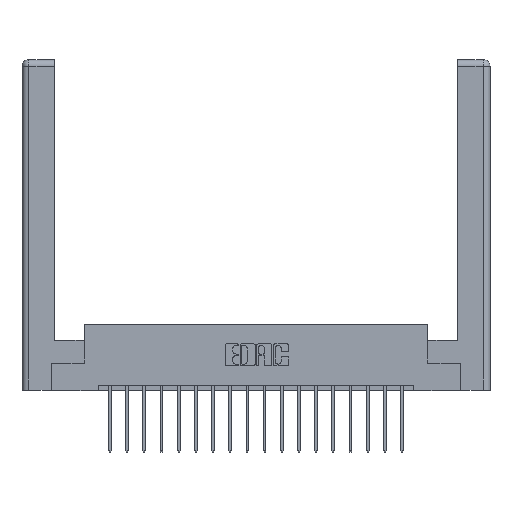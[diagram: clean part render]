
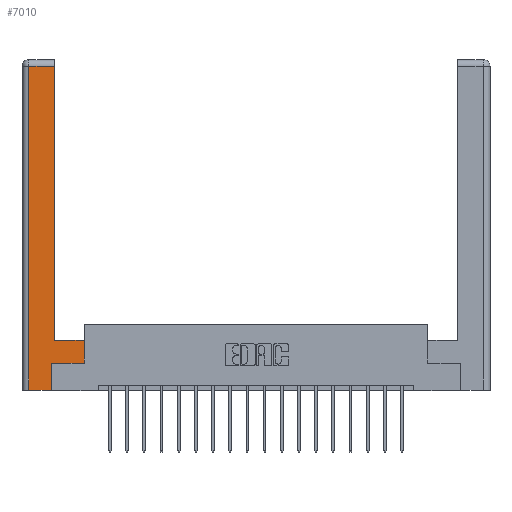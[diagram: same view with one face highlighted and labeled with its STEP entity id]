
A CAD part, top view. The second image highlights one B-rep face of the part: STEP entity #7010.
In plain terms, the highlighted planar face has unit normal (0, 0, 1).
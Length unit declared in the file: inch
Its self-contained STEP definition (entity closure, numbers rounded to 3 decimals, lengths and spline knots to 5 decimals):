
#259 = ORIENTED_EDGE ( 'NONE', *, *, #2643, .T. ) ;
#752 = DIRECTION ( 'NONE',  ( -1., 0., 0. ) ) ;
#872 = CARTESIAN_POINT ( 'NONE',  ( 0.565, 0.245, 0. ) ) ;
#1213 = VECTOR ( 'NONE', #17322, 39.37008 ) ;
#1403 = CARTESIAN_POINT ( 'NONE',  ( 0.265, 0.245, 0. ) ) ;
#1741 = LINE ( 'NONE', #13381, #9340 ) ;
#1942 = VERTEX_POINT ( 'NONE', #7242 ) ;
#1962 = EDGE_CURVE ( 'NONE', #15366, #17851, #3437, .T. ) ;
#2643 = EDGE_CURVE ( 'NONE', #3996, #12572, #1741, .T. ) ;
#3410 = LINE ( 'NONE', #872, #1213 ) ;
#3437 = LINE ( 'NONE', #14889, #15079 ) ;
#3588 = ORIENTED_EDGE ( 'NONE', *, *, #8873, .T. ) ;
#3723 = LINE ( 'NONE', #14068, #6114 ) ;
#3759 = CARTESIAN_POINT ( 'NONE',  ( 0.565, 0.245, 0. ) ) ;
#3996 = VERTEX_POINT ( 'NONE', #14719 ) ;
#5670 = ORIENTED_EDGE ( 'NONE', *, *, #1962, .T. ) ;
#5681 = LINE ( 'NONE', #6762, #17355 ) ;
#5781 = DIRECTION ( 'NONE',  ( 0., 1., 0. ) ) ;
#5881 = EDGE_CURVE ( 'NONE', #15811, #10688, #11456, .T. ) ;
#6114 = VECTOR ( 'NONE', #752, 39.37008 ) ;
#6762 = CARTESIAN_POINT ( 'NONE',  ( 0.295, 0.45, 0. ) ) ;
#6776 = CARTESIAN_POINT ( 'NONE',  ( 0.565, 0.45, 0. ) ) ;
#6832 = EDGE_CURVE ( 'NONE', #10688, #15366, #5681, .T. ) ;
#6888 = DIRECTION ( 'NONE',  ( -1., 0., 0. ) ) ;
#7006 = PLANE ( 'NONE',  #16360 ) ;
#7010 = ADVANCED_FACE ( 'NONE', ( #18062 ), #7006, .F. ) ;
#7195 = DIRECTION ( 'NONE',  ( 0., 1., 0. ) ) ;
#7242 = CARTESIAN_POINT ( 'NONE',  ( 0.265, 0.245, 0. ) ) ;
#7740 = CARTESIAN_POINT ( 'NONE',  ( 0.295, 2.94, 0. ) ) ;
#7764 = CARTESIAN_POINT ( 'NONE',  ( 0.295, 0.45, 0. ) ) ;
#8056 = EDGE_CURVE ( 'NONE', #17851, #3996, #3723, .T. ) ;
#8361 = VECTOR ( 'NONE', #18960, 39.37008 ) ;
#8441 = EDGE_LOOP ( 'NONE', ( #5670, #14473, #259, #9041, #13073, #3588, #11822, #15148 ) ) ;
#8710 = DIRECTION ( 'NONE',  ( 0., -1., 0. ) ) ;
#8873 = EDGE_CURVE ( 'NONE', #1942, #15811, #3410, .T. ) ;
#9041 = ORIENTED_EDGE ( 'NONE', *, *, #18724, .T. ) ;
#9109 = CARTESIAN_POINT ( 'NONE',  ( 0.265, 0., 0. ) ) ;
#9340 = VECTOR ( 'NONE', #8710, 39.37008 ) ;
#9548 = CARTESIAN_POINT ( 'NONE',  ( 0.0615, 0., 0. ) ) ;
#10074 = CARTESIAN_POINT ( 'NONE',  ( 0.565, 0.45, 0. ) ) ;
#10300 = DIRECTION ( 'NONE',  ( 1., 0., 0. ) ) ;
#10688 = VERTEX_POINT ( 'NONE', #10074 ) ;
#11192 = VECTOR ( 'NONE', #7195, 39.37008 ) ;
#11456 = LINE ( 'NONE', #6776, #8361 ) ;
#11822 = ORIENTED_EDGE ( 'NONE', *, *, #5881, .T. ) ;
#12572 = VERTEX_POINT ( 'NONE', #9548 ) ;
#12860 = VERTEX_POINT ( 'NONE', #9109 ) ;
#13067 = DIRECTION ( 'NONE',  ( 0., 0., -1. ) ) ;
#13073 = ORIENTED_EDGE ( 'NONE', *, *, #19623, .T. ) ;
#13323 = CARTESIAN_POINT ( 'NONE',  ( 0., 0., 0. ) ) ;
#13381 = CARTESIAN_POINT ( 'NONE',  ( 0.0615, 0., 0. ) ) ;
#14068 = CARTESIAN_POINT ( 'NONE',  ( 0.0615, 2.94, 0. ) ) ;
#14473 = ORIENTED_EDGE ( 'NONE', *, *, #8056, .T. ) ;
#14719 = CARTESIAN_POINT ( 'NONE',  ( 0.0615, 2.94, 0. ) ) ;
#14889 = CARTESIAN_POINT ( 'NONE',  ( 0.295, 3., 0. ) ) ;
#15033 = LINE ( 'NONE', #16158, #15757 ) ;
#15079 = VECTOR ( 'NONE', #5781, 39.37008 ) ;
#15148 = ORIENTED_EDGE ( 'NONE', *, *, #6832, .T. ) ;
#15366 = VERTEX_POINT ( 'NONE', #7764 ) ;
#15757 = VECTOR ( 'NONE', #10300, 39.37008 ) ;
#15811 = VERTEX_POINT ( 'NONE', #3759 ) ;
#16158 = CARTESIAN_POINT ( 'NONE',  ( 0.265, 0., 0. ) ) ;
#16360 = AXIS2_PLACEMENT_3D ( 'NONE', #13323, #13067, #16372 ) ;
#16372 = DIRECTION ( 'NONE',  ( -1., 0., 0. ) ) ;
#17322 = DIRECTION ( 'NONE',  ( 1., 0., 0. ) ) ;
#17355 = VECTOR ( 'NONE', #6888, 39.37008 ) ;
#17851 = VERTEX_POINT ( 'NONE', #7740 ) ;
#18062 = FACE_OUTER_BOUND ( 'NONE', #8441, .T. ) ;
#18724 = EDGE_CURVE ( 'NONE', #12572, #12860, #15033, .T. ) ;
#18825 = LINE ( 'NONE', #1403, #11192 ) ;
#18960 = DIRECTION ( 'NONE',  ( 0., 1., 0. ) ) ;
#19623 = EDGE_CURVE ( 'NONE', #12860, #1942, #18825, .T. ) ;
